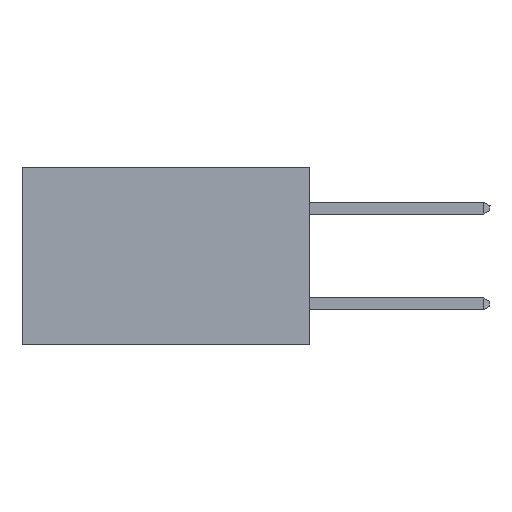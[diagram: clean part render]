
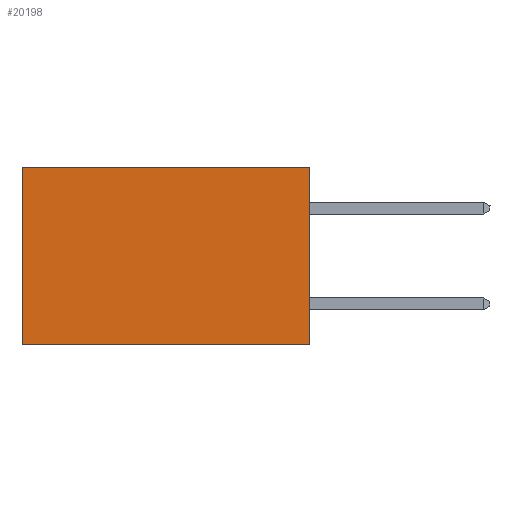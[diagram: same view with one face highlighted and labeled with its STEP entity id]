
A CAD part, left-side view. The second image highlights one B-rep face of the part: STEP entity #20198.
In plain terms, the highlighted planar face has unit normal (-1, 0, 0).
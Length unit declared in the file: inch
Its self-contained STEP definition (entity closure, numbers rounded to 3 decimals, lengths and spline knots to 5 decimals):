
#787 = VECTOR ( 'NONE', #14911, 39.37008 ) ;
#1661 = LINE ( 'NONE', #14454, #787 ) ;
#1732 = ORIENTED_EDGE ( 'NONE', *, *, #8684, .T. ) ;
#1882 = AXIS2_PLACEMENT_3D ( 'NONE', #9567, #4165, #20652 ) ;
#4165 = DIRECTION ( 'NONE',  ( 1., 0., 0. ) ) ;
#6468 = DIRECTION ( 'NONE',  ( 0., 0., -1. ) ) ;
#6510 = VERTEX_POINT ( 'NONE', #14318 ) ;
#7950 = LINE ( 'NONE', #10152, #20459 ) ;
#8135 = FACE_OUTER_BOUND ( 'NONE', #14035, .T. ) ;
#8684 = EDGE_CURVE ( 'NONE', #11963, #6510, #7950, .T. ) ;
#8766 = VERTEX_POINT ( 'NONE', #19635 ) ;
#8925 = EDGE_CURVE ( 'NONE', #6510, #17218, #1661, .T. ) ;
#9567 = CARTESIAN_POINT ( 'NONE',  ( 0.2875, 0., 0. ) ) ;
#10092 = CARTESIAN_POINT ( 'NONE',  ( 0.2875, 0., 0. ) ) ;
#10152 = CARTESIAN_POINT ( 'NONE',  ( 0.2875, 0., 0. ) ) ;
#11812 = ORIENTED_EDGE ( 'NONE', *, *, #21593, .F. ) ;
#11963 = VERTEX_POINT ( 'NONE', #10092 ) ;
#13249 = CARTESIAN_POINT ( 'NONE',  ( 0.2875, 0., -0.37 ) ) ;
#13936 = LINE ( 'NONE', #13249, #19948 ) ;
#14035 = EDGE_LOOP ( 'NONE', ( #17244, #20538, #11812, #1732 ) ) ;
#14318 = CARTESIAN_POINT ( 'NONE',  ( 0.2875, 0.6, 0. ) ) ;
#14454 = CARTESIAN_POINT ( 'NONE',  ( 0.2875, 0.6, 0. ) ) ;
#14752 = PLANE ( 'NONE',  #1882 ) ;
#14911 = DIRECTION ( 'NONE',  ( 0., 0., -1. ) ) ;
#15117 = VECTOR ( 'NONE', #6468, 39.37008 ) ;
#16063 = EDGE_CURVE ( 'NONE', #8766, #17218, #13936, .T. ) ;
#17218 = VERTEX_POINT ( 'NONE', #22608 ) ;
#17244 = ORIENTED_EDGE ( 'NONE', *, *, #8925, .T. ) ;
#18606 = DIRECTION ( 'NONE',  ( 0., 1., 0. ) ) ;
#19635 = CARTESIAN_POINT ( 'NONE',  ( 0.2875, 0., -0.37 ) ) ;
#19948 = VECTOR ( 'NONE', #18606, 39.37008 ) ;
#20040 = LINE ( 'NONE', #22777, #15117 ) ;
#20198 = ADVANCED_FACE ( 'NONE', ( #8135 ), #14752, .F. ) ;
#20459 = VECTOR ( 'NONE', #22910, 39.37008 ) ;
#20538 = ORIENTED_EDGE ( 'NONE', *, *, #16063, .F. ) ;
#20652 = DIRECTION ( 'NONE',  ( 0., 0., -1. ) ) ;
#21593 = EDGE_CURVE ( 'NONE', #11963, #8766, #20040, .T. ) ;
#22608 = CARTESIAN_POINT ( 'NONE',  ( 0.2875, 0.6, -0.37 ) ) ;
#22777 = CARTESIAN_POINT ( 'NONE',  ( 0.2875, 0., 0. ) ) ;
#22910 = DIRECTION ( 'NONE',  ( 0., 1., 0. ) ) ;
